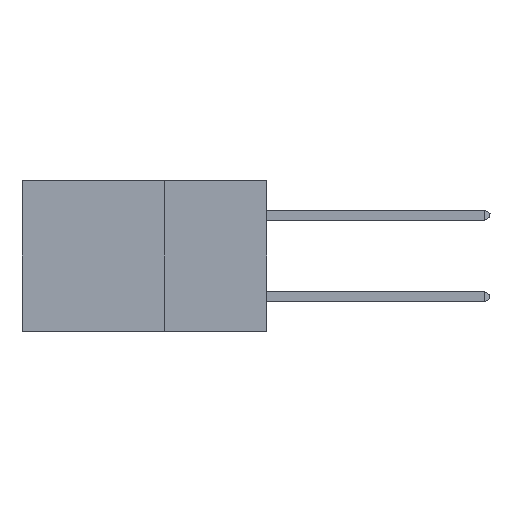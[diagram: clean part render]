
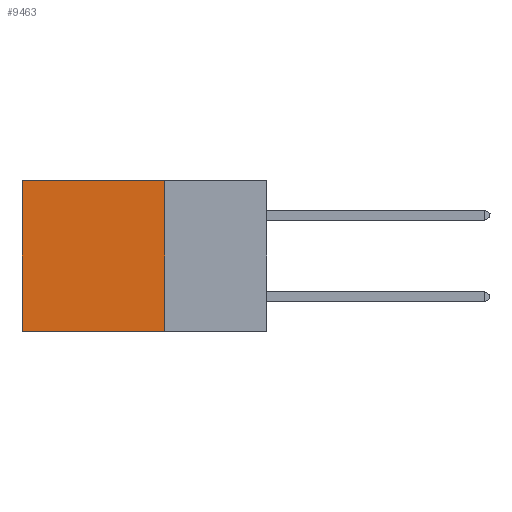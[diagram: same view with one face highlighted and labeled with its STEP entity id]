
A CAD part, left-side view. The second image highlights one B-rep face of the part: STEP entity #9463.
In plain terms, the highlighted planar face has unit normal (-1, 0, 0).
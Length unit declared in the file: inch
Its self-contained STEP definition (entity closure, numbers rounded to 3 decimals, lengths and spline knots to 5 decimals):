
#2349 = CARTESIAN_POINT ( 'NONE',  ( 0.2875, 0.6, -0.37 ) ) ;
#2991 = DIRECTION ( 'NONE',  ( 0., 0., -1. ) ) ;
#3046 = VECTOR ( 'NONE', #11291, 39.37008 ) ;
#4226 = LINE ( 'NONE', #25587, #25608 ) ;
#6907 = EDGE_CURVE ( 'NONE', #24503, #7873, #36685, .T. ) ;
#7873 = VERTEX_POINT ( 'NONE', #22169 ) ;
#8385 = VERTEX_POINT ( 'NONE', #9254 ) ;
#8474 = EDGE_CURVE ( 'NONE', #8385, #10812, #28500, .T. ) ;
#8732 = DIRECTION ( 'NONE',  ( 0., 0., -1. ) ) ;
#9254 = CARTESIAN_POINT ( 'NONE',  ( 0.2875, 0.25, -0.37 ) ) ;
#9463 = ADVANCED_FACE ( 'NONE', ( #40102 ), #24380, .F. ) ;
#10812 = VERTEX_POINT ( 'NONE', #2349 ) ;
#10851 = CARTESIAN_POINT ( 'NONE',  ( 0.2875, 0.6, 0. ) ) ;
#11291 = DIRECTION ( 'NONE',  ( 0., 0., -1. ) ) ;
#11576 = CARTESIAN_POINT ( 'NONE',  ( 0.2875, 0.25, 0. ) ) ;
#11825 = VECTOR ( 'NONE', #31040, 39.37008 ) ;
#12302 = EDGE_CURVE ( 'NONE', #7873, #10812, #26896, .T. ) ;
#18416 = CARTESIAN_POINT ( 'NONE',  ( 0.2875, 0.25, 0. ) ) ;
#18842 = CARTESIAN_POINT ( 'NONE',  ( 0.2875, 0.25, -0.37 ) ) ;
#21308 = ORIENTED_EDGE ( 'NONE', *, *, #12302, .T. ) ;
#22169 = CARTESIAN_POINT ( 'NONE',  ( 0.2875, 0.6, 0. ) ) ;
#24380 = PLANE ( 'NONE',  #32153 ) ;
#24503 = VERTEX_POINT ( 'NONE', #37100 ) ;
#25587 = CARTESIAN_POINT ( 'NONE',  ( 0.2875, 0.25, 0. ) ) ;
#25608 = VECTOR ( 'NONE', #2991, 39.37008 ) ;
#26896 = LINE ( 'NONE', #10851, #3046 ) ;
#27499 = VECTOR ( 'NONE', #30595, 39.37008 ) ;
#28500 = LINE ( 'NONE', #18842, #27499 ) ;
#28683 = ORIENTED_EDGE ( 'NONE', *, *, #6907, .T. ) ;
#30501 = EDGE_CURVE ( 'NONE', #24503, #8385, #4226, .T. ) ;
#30595 = DIRECTION ( 'NONE',  ( 0., 1., 0. ) ) ;
#31040 = DIRECTION ( 'NONE',  ( 0., 1., 0. ) ) ;
#32153 = AXIS2_PLACEMENT_3D ( 'NONE', #11576, #34235, #8732 ) ;
#33935 = ORIENTED_EDGE ( 'NONE', *, *, #8474, .F. ) ;
#34235 = DIRECTION ( 'NONE',  ( 1., 0., 0. ) ) ;
#36685 = LINE ( 'NONE', #18416, #11825 ) ;
#37100 = CARTESIAN_POINT ( 'NONE',  ( 0.2875, 0.25, 0. ) ) ;
#39356 = ORIENTED_EDGE ( 'NONE', *, *, #30501, .F. ) ;
#40102 = FACE_OUTER_BOUND ( 'NONE', #41694, .T. ) ;
#41694 = EDGE_LOOP ( 'NONE', ( #21308, #33935, #39356, #28683 ) ) ;
